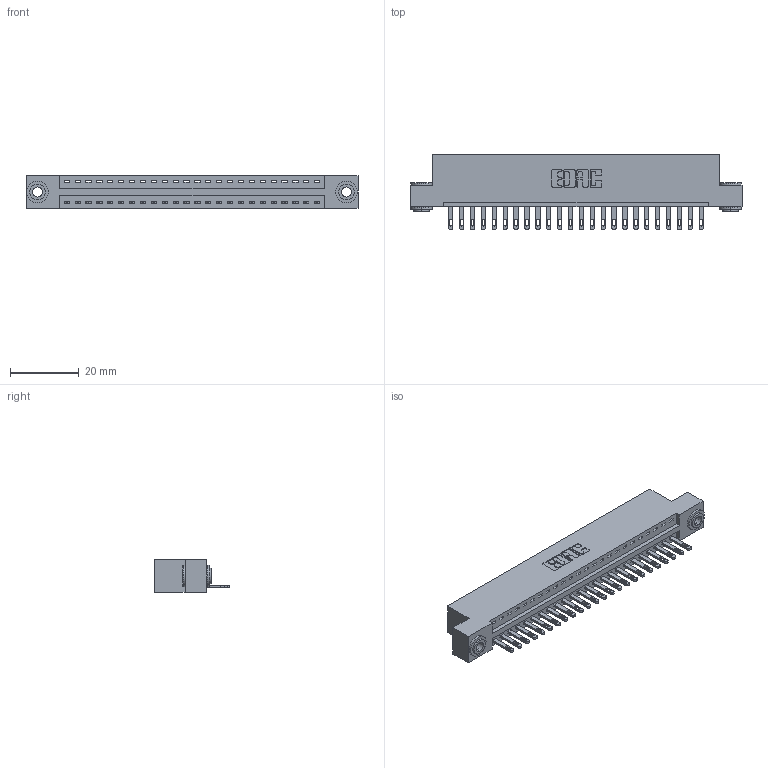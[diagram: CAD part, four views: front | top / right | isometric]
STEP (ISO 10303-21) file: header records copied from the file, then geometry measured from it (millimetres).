
FILE_DESCRIPTION (( 'STEP AP203' ), '1' );
FILE_NAME ('346-024-500-103.STEP', '2022-05-05T22:06:21', ( '' ), ( '' ), 'SwSTEP 2.0', 'SolidWorks 2020', '' );
FILE_SCHEMA (( 'CONFIG_CONTROL_DESIGN' ));
Length unit declared in the file: inch
Products named in the file (4): 345-292-001_345-293-100; 345-250-002_345-250-002-102; 346-024-500-103; 346 Part_Flush Mounting Lugs - 0.156 Dia-TH
Assembly tree (27 placements, depth 2):
  346-024-500-103
    346 Part_Flush Mounting Lugs - 0.156 Dia-TH
    345-292-001_345-293-100  x24
    345-250-002_345-250-002-102  x2
Bounding box: 96.77 x 21.84 x 9.4 mm (x, y, z)
Volume: 9155.5 mm3; surface area: 11556.4 mm2
Topology: 27 solids, 27 shells, 1470 faces, 4473 edges, 2978 vertices
Faces by surface type: plane 916, cylinder 546, cone 8
Entity records: 18314 total; most frequent: CARTESIAN_POINT 3125, ORIENTED_EDGE 3074, DIRECTION 2811, EDGE_CURVE 1537, LINE 1281, VECTOR 1281, VERTEX_POINT 1022, AXIS2_PLACEMENT_3D 765
